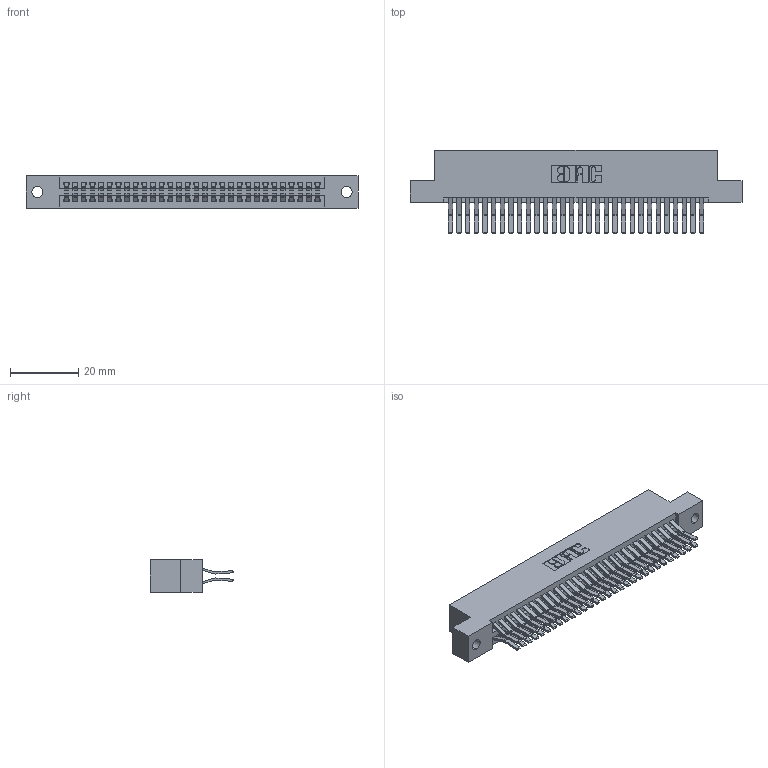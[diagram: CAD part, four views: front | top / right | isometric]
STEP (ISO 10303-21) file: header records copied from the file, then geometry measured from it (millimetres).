
FILE_DESCRIPTION (( 'STEP AP203' ), '1' );
FILE_NAME ('395-060-560-202.STEP', '2019-10-23T15:09:53', ( '' ), ( '' ), 'SwSTEP 2.0', 'SolidWorks 2016', '' );
FILE_SCHEMA (( 'CONFIG_CONTROL_DESIGN' ));
Length unit declared in the file: inch
Products named in the file (3): 345-292-001_560 Tail; 395-060-560-202; 345 Part_Flush Mounting Lugs - 0.128 Dia
Assembly tree (61 placements, depth 2):
  395-060-560-202
    345 Part_Flush Mounting Lugs - 0.128 Dia
    345-292-001_560 Tail  x60
Bounding box: 97.41 x 24.45 x 9.4 mm (x, y, z)
Volume: 9707.6 mm3; surface area: 14855.8 mm2
Topology: 61 solids, 61 shells, 3246 faces, 9641 edges, 6346 vertices
Faces by surface type: plane 2060, cylinder 1186
Entity records: 25245 total; most frequent: CARTESIAN_POINT 4244, ORIENTED_EDGE 4178, DIRECTION 3761, EDGE_CURVE 2089, LINE 1833, VECTOR 1833, VERTEX_POINT 1390, AXIS2_PLACEMENT_3D 964
